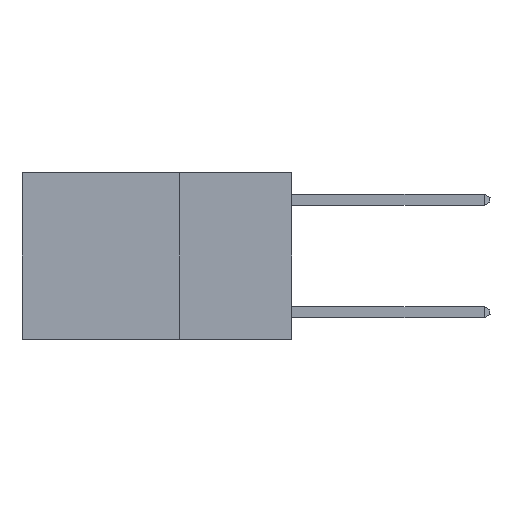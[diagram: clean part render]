
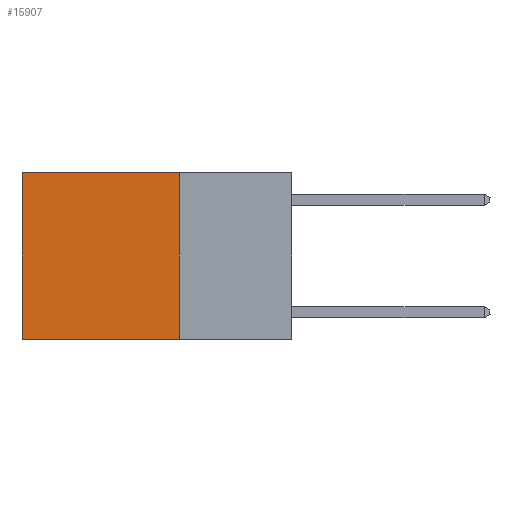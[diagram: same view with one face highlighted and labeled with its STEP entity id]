
A CAD part, left-side view. The second image highlights one B-rep face of the part: STEP entity #15907.
In plain terms, the highlighted planar face has unit normal (-1, 0, 0).
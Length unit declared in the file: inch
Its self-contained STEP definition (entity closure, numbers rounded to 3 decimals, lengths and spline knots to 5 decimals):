
#200 = CARTESIAN_POINT ( 'NONE',  ( 0.2625, 0.6, -0.37 ) ) ;
#1118 = DIRECTION ( 'NONE',  ( 0., 0., -1. ) ) ;
#1157 = CARTESIAN_POINT ( 'NONE',  ( 0.2625, 0.6, 0. ) ) ;
#1664 = LINE ( 'NONE', #23644, #2658 ) ;
#1794 = VERTEX_POINT ( 'NONE', #1157 ) ;
#2106 = CARTESIAN_POINT ( 'NONE',  ( 0.2625, 0.25, 0. ) ) ;
#2658 = VECTOR ( 'NONE', #5153, 39.37008 ) ;
#2678 = DIRECTION ( 'NONE',  ( 0., 0., -1. ) ) ;
#4525 = VECTOR ( 'NONE', #18513, 39.37008 ) ;
#5153 = DIRECTION ( 'NONE',  ( 0., 1., 0. ) ) ;
#6374 = CARTESIAN_POINT ( 'NONE',  ( 0.2625, 0.25, -0.37 ) ) ;
#6873 = LINE ( 'NONE', #10564, #8310 ) ;
#7354 = EDGE_LOOP ( 'NONE', ( #9084, #19286, #11376, #17419 ) ) ;
#8310 = VECTOR ( 'NONE', #1118, 39.37008 ) ;
#9084 = ORIENTED_EDGE ( 'NONE', *, *, #12934, .T. ) ;
#9308 = CARTESIAN_POINT ( 'NONE',  ( 0.2625, 0.25, 0. ) ) ;
#9514 = EDGE_CURVE ( 'NONE', #22129, #23648, #10204, .T. ) ;
#9752 = PLANE ( 'NONE',  #12872 ) ;
#10204 = LINE ( 'NONE', #6374, #10893 ) ;
#10564 = CARTESIAN_POINT ( 'NONE',  ( 0.2625, 0.6, 0. ) ) ;
#10893 = VECTOR ( 'NONE', #17280, 39.37008 ) ;
#11376 = ORIENTED_EDGE ( 'NONE', *, *, #14050, .F. ) ;
#11524 = EDGE_CURVE ( 'NONE', #14178, #1794, #1664, .T. ) ;
#12076 = CARTESIAN_POINT ( 'NONE',  ( 0.2625, 0.25, -0.37 ) ) ;
#12139 = DIRECTION ( 'NONE',  ( 1., 0., 0. ) ) ;
#12872 = AXIS2_PLACEMENT_3D ( 'NONE', #15483, #12139, #2678 ) ;
#12934 = EDGE_CURVE ( 'NONE', #1794, #23648, #6873, .T. ) ;
#14050 = EDGE_CURVE ( 'NONE', #14178, #22129, #16614, .T. ) ;
#14178 = VERTEX_POINT ( 'NONE', #9308 ) ;
#15483 = CARTESIAN_POINT ( 'NONE',  ( 0.2625, 0.25, 0. ) ) ;
#15907 = ADVANCED_FACE ( 'NONE', ( #18850 ), #9752, .F. ) ;
#16614 = LINE ( 'NONE', #2106, #4525 ) ;
#17280 = DIRECTION ( 'NONE',  ( 0., 1., 0. ) ) ;
#17419 = ORIENTED_EDGE ( 'NONE', *, *, #11524, .T. ) ;
#18513 = DIRECTION ( 'NONE',  ( 0., 0., -1. ) ) ;
#18850 = FACE_OUTER_BOUND ( 'NONE', #7354, .T. ) ;
#19286 = ORIENTED_EDGE ( 'NONE', *, *, #9514, .F. ) ;
#22129 = VERTEX_POINT ( 'NONE', #12076 ) ;
#23644 = CARTESIAN_POINT ( 'NONE',  ( 0.2625, 0.25, 0. ) ) ;
#23648 = VERTEX_POINT ( 'NONE', #200 ) ;
